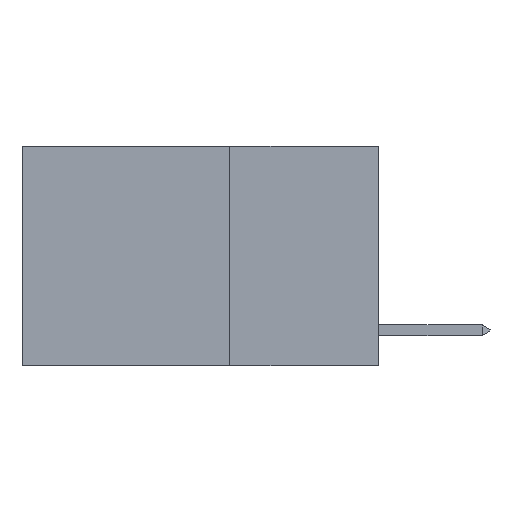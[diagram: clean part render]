
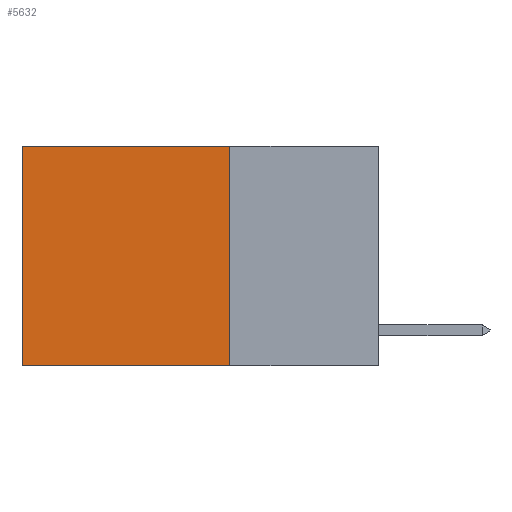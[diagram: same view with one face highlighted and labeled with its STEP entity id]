
A CAD part, left-side view. The second image highlights one B-rep face of the part: STEP entity #5632.
In plain terms, the highlighted planar face has unit normal (-1, 0, 0).
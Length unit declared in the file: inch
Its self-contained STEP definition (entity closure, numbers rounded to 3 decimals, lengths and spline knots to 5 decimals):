
#217 = EDGE_LOOP ( 'NONE', ( #11228, #11989, #6823, #10768 ) ) ;
#1162 = EDGE_CURVE ( 'NONE', #8034, #3244, #3679, .T. ) ;
#1477 = VECTOR ( 'NONE', #7575, 39.37008 ) ;
#2535 = PLANE ( 'NONE',  #8129 ) ;
#2590 = DIRECTION ( 'NONE',  ( 1., 0., 0. ) ) ;
#3051 = CARTESIAN_POINT ( 'NONE',  ( 0.2625, 0.6, -0.37 ) ) ;
#3152 = EDGE_CURVE ( 'NONE', #3244, #4214, #4617, .T. ) ;
#3244 = VERTEX_POINT ( 'NONE', #6541 ) ;
#3608 = CARTESIAN_POINT ( 'NONE',  ( 0.2625, 0.25, 0. ) ) ;
#3679 = LINE ( 'NONE', #12824, #11269 ) ;
#4214 = VERTEX_POINT ( 'NONE', #3051 ) ;
#4489 = DIRECTION ( 'NONE',  ( 0., 0., -1. ) ) ;
#4617 = LINE ( 'NONE', #7563, #1477 ) ;
#4732 = CARTESIAN_POINT ( 'NONE',  ( 0.2625, 0.25, 0. ) ) ;
#5136 = VERTEX_POINT ( 'NONE', #9796 ) ;
#5242 = LINE ( 'NONE', #5993, #5553 ) ;
#5338 = VECTOR ( 'NONE', #12155, 39.37008 ) ;
#5553 = VECTOR ( 'NONE', #7075, 39.37008 ) ;
#5632 = ADVANCED_FACE ( 'NONE', ( #12717 ), #2535, .F. ) ;
#5993 = CARTESIAN_POINT ( 'NONE',  ( 0.2625, 0.25, 0. ) ) ;
#6315 = CARTESIAN_POINT ( 'NONE',  ( 0.2625, 0.6, 0. ) ) ;
#6541 = CARTESIAN_POINT ( 'NONE',  ( 0.2625, 0.25, -0.37 ) ) ;
#6823 = ORIENTED_EDGE ( 'NONE', *, *, #1162, .F. ) ;
#7075 = DIRECTION ( 'NONE',  ( 0., 1., 0. ) ) ;
#7563 = CARTESIAN_POINT ( 'NONE',  ( 0.2625, 0.25, -0.37 ) ) ;
#7575 = DIRECTION ( 'NONE',  ( 0., 1., 0. ) ) ;
#8034 = VERTEX_POINT ( 'NONE', #4732 ) ;
#8129 = AXIS2_PLACEMENT_3D ( 'NONE', #3608, #2590, #9607 ) ;
#8640 = EDGE_CURVE ( 'NONE', #8034, #5136, #5242, .T. ) ;
#9607 = DIRECTION ( 'NONE',  ( 0., 0., -1. ) ) ;
#9796 = CARTESIAN_POINT ( 'NONE',  ( 0.2625, 0.6, 0. ) ) ;
#10217 = LINE ( 'NONE', #6315, #5338 ) ;
#10768 = ORIENTED_EDGE ( 'NONE', *, *, #8640, .T. ) ;
#11025 = EDGE_CURVE ( 'NONE', #5136, #4214, #10217, .T. ) ;
#11228 = ORIENTED_EDGE ( 'NONE', *, *, #11025, .T. ) ;
#11269 = VECTOR ( 'NONE', #4489, 39.37008 ) ;
#11989 = ORIENTED_EDGE ( 'NONE', *, *, #3152, .F. ) ;
#12155 = DIRECTION ( 'NONE',  ( 0., 0., -1. ) ) ;
#12717 = FACE_OUTER_BOUND ( 'NONE', #217, .T. ) ;
#12824 = CARTESIAN_POINT ( 'NONE',  ( 0.2625, 0.25, 0. ) ) ;
